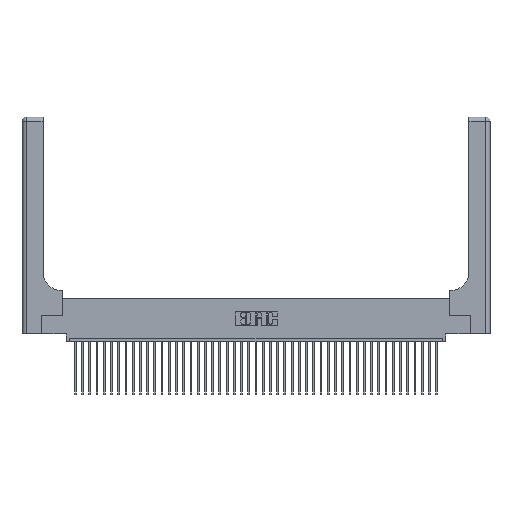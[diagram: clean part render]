
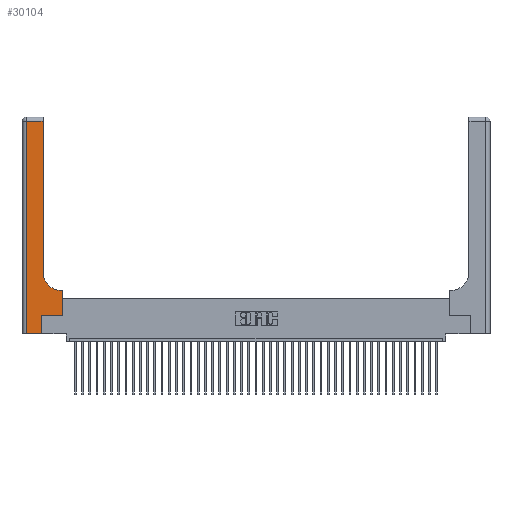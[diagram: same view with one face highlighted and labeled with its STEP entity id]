
A CAD part, top view. The second image highlights one B-rep face of the part: STEP entity #30104.
In plain terms, the highlighted planar face has unit normal (0, 0, 1).
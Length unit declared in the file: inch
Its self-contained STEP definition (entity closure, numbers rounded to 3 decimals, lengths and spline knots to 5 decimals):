
#542 = EDGE_CURVE ( 'NONE', #16153, #23807, #18232, .T. ) ;
#1547 = CARTESIAN_POINT ( 'NONE',  ( 0.06, 2.94, 0.37 ) ) ;
#2321 = CIRCLE ( 'NONE', #33472, 0.25 ) ;
#3397 = DIRECTION ( 'NONE',  ( 0., 1., 0. ) ) ;
#4337 = LINE ( 'NONE', #27286, #33545 ) ;
#6256 = VERTEX_POINT ( 'NONE', #41053 ) ;
#6328 = ORIENTED_EDGE ( 'NONE', *, *, #35631, .T. ) ;
#6386 = DIRECTION ( 'NONE',  ( -1., 0., 0. ) ) ;
#6438 = DIRECTION ( 'NONE',  ( 1., 0., 0. ) ) ;
#6924 = VERTEX_POINT ( 'NONE', #19651 ) ;
#7135 = EDGE_CURVE ( 'NONE', #37070, #16153, #39434, .T. ) ;
#7893 = VECTOR ( 'NONE', #6438, 39.37008 ) ;
#9034 = VECTOR ( 'NONE', #37523, 39.37008 ) ;
#9123 = VECTOR ( 'NONE', #9567, 39.37008 ) ;
#9567 = DIRECTION ( 'NONE',  ( 1., 0., 0. ) ) ;
#12093 = ORIENTED_EDGE ( 'NONE', *, *, #42506, .T. ) ;
#12230 = EDGE_CURVE ( 'NONE', #26653, #33638, #29627, .T. ) ;
#12249 = CARTESIAN_POINT ( 'NONE',  ( 0.06, 3., 0.37 ) ) ;
#12621 = VECTOR ( 'NONE', #22010, 39.37008 ) ;
#13155 = ORIENTED_EDGE ( 'NONE', *, *, #17926, .T. ) ;
#13170 = CARTESIAN_POINT ( 'NONE',  ( 0.5585, 0.25, 0.37 ) ) ;
#14400 = DIRECTION ( 'NONE',  ( 0., 1., 0. ) ) ;
#15338 = ORIENTED_EDGE ( 'NONE', *, *, #542, .T. ) ;
#15396 = CARTESIAN_POINT ( 'NONE',  ( 0.5415, 0.85, 0.37 ) ) ;
#15575 = ORIENTED_EDGE ( 'NONE', *, *, #41451, .T. ) ;
#16021 = CARTESIAN_POINT ( 'NONE',  ( 0., 3., 0.37 ) ) ;
#16153 = VERTEX_POINT ( 'NONE', #29177 ) ;
#16214 = LINE ( 'NONE', #12249, #12621 ) ;
#16230 = DIRECTION ( 'NONE',  ( -1., 0., 0. ) ) ;
#16674 = CARTESIAN_POINT ( 'NONE',  ( 0.269, 0., 0.37 ) ) ;
#17926 = EDGE_CURVE ( 'NONE', #30538, #39605, #16214, .T. ) ;
#18232 = LINE ( 'NONE', #40189, #29488 ) ;
#18708 = LINE ( 'NONE', #39355, #7893 ) ;
#19105 = ORIENTED_EDGE ( 'NONE', *, *, #12230, .T. ) ;
#19264 = ORIENTED_EDGE ( 'NONE', *, *, #24039, .T. ) ;
#19651 = CARTESIAN_POINT ( 'NONE',  ( 0.2915, 2.94, 0.37 ) ) ;
#22010 = DIRECTION ( 'NONE',  ( 0., -1., 0. ) ) ;
#22061 = VECTOR ( 'NONE', #3397, 39.37008 ) ;
#23175 = CARTESIAN_POINT ( 'NONE',  ( 0.5585, 0.25, 0.37 ) ) ;
#23807 = VERTEX_POINT ( 'NONE', #34297 ) ;
#24039 = EDGE_CURVE ( 'NONE', #23807, #6256, #2321, .T. ) ;
#24247 = ORIENTED_EDGE ( 'NONE', *, *, #35387, .T. ) ;
#24965 = CARTESIAN_POINT ( 'NONE',  ( 0.269, 0.25, 0.37 ) ) ;
#25814 = DIRECTION ( 'NONE',  ( 0., 0., -1. ) ) ;
#26653 = VERTEX_POINT ( 'NONE', #30341 ) ;
#27286 = CARTESIAN_POINT ( 'NONE',  ( 0.2915, 3., 0.37 ) ) ;
#28688 = DIRECTION ( 'NONE',  ( 1., 0., 0. ) ) ;
#28766 = DIRECTION ( 'NONE',  ( 0., 0., -1. ) ) ;
#29176 = CARTESIAN_POINT ( 'NONE',  ( 0.269, 0.25, 0.37 ) ) ;
#29177 = CARTESIAN_POINT ( 'NONE',  ( 0.5585, 0.6, 0.37 ) ) ;
#29488 = VECTOR ( 'NONE', #16230, 39.37008 ) ;
#29627 = LINE ( 'NONE', #16674, #36725 ) ;
#29639 = AXIS2_PLACEMENT_3D ( 'NONE', #16021, #28766, #6386 ) ;
#30104 = ADVANCED_FACE ( 'NONE', ( #34117 ), #32286, .F. ) ;
#30341 = CARTESIAN_POINT ( 'NONE',  ( 0.269, 0., 0.37 ) ) ;
#30538 = VERTEX_POINT ( 'NONE', #1547 ) ;
#32286 = PLANE ( 'NONE',  #29639 ) ;
#32559 = LINE ( 'NONE', #37377, #9034 ) ;
#33472 = AXIS2_PLACEMENT_3D ( 'NONE', #15396, #25814, #28688 ) ;
#33545 = VECTOR ( 'NONE', #14400, 39.37008 ) ;
#33638 = VERTEX_POINT ( 'NONE', #24965 ) ;
#33788 = DIRECTION ( 'NONE',  ( 0., 1., 0. ) ) ;
#34117 = FACE_OUTER_BOUND ( 'NONE', #42220, .T. ) ;
#34297 = CARTESIAN_POINT ( 'NONE',  ( 0.5415, 0.6, 0.37 ) ) ;
#35232 = LINE ( 'NONE', #29176, #9123 ) ;
#35387 = EDGE_CURVE ( 'NONE', #39605, #26653, #18708, .T. ) ;
#35631 = EDGE_CURVE ( 'NONE', #6256, #6924, #4337, .T. ) ;
#36091 = CARTESIAN_POINT ( 'NONE',  ( 0.06, 0., 0.37 ) ) ;
#36725 = VECTOR ( 'NONE', #33788, 39.37008 ) ;
#37070 = VERTEX_POINT ( 'NONE', #13170 ) ;
#37377 = CARTESIAN_POINT ( 'NONE',  ( 0., 2.94, 0.37 ) ) ;
#37523 = DIRECTION ( 'NONE',  ( -1., 0., 0. ) ) ;
#39355 = CARTESIAN_POINT ( 'NONE',  ( 0., 0., 0.37 ) ) ;
#39434 = LINE ( 'NONE', #23175, #22061 ) ;
#39605 = VERTEX_POINT ( 'NONE', #36091 ) ;
#40189 = CARTESIAN_POINT ( 'NONE',  ( 0.2915, 0.6, 0.37 ) ) ;
#41053 = CARTESIAN_POINT ( 'NONE',  ( 0.2915, 0.85, 0.37 ) ) ;
#41254 = ORIENTED_EDGE ( 'NONE', *, *, #7135, .T. ) ;
#41451 = EDGE_CURVE ( 'NONE', #33638, #37070, #35232, .T. ) ;
#42220 = EDGE_LOOP ( 'NONE', ( #6328, #12093, #13155, #24247, #19105, #15575, #41254, #15338, #19264 ) ) ;
#42506 = EDGE_CURVE ( 'NONE', #6924, #30538, #32559, .T. ) ;
